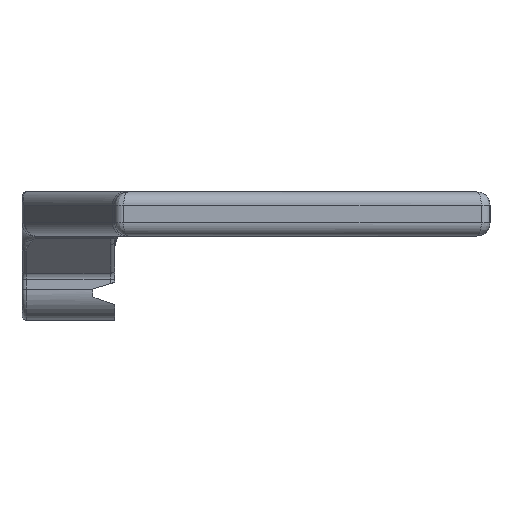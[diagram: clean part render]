
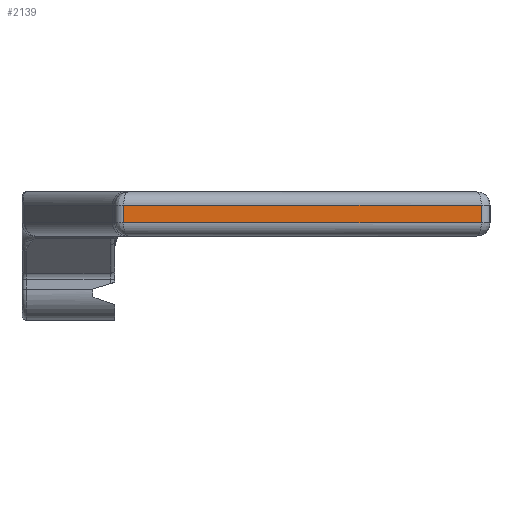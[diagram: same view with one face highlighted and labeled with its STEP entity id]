
A CAD part, left-side view. The second image highlights one B-rep face of the part: STEP entity #2139.
In plain terms, the highlighted planar face has unit normal (-1, 0, 0).
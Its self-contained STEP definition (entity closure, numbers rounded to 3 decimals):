
#67=PLANE('',#2383);
#225=FACE_OUTER_BOUND('',#368,.T.);
#368=EDGE_LOOP('',(#1737,#1738,#1739,#1740));
#515=LINE('',#4032,#679);
#524=LINE('',#4059,#688);
#525=LINE('',#4063,#689);
#526=LINE('',#4064,#690);
#679=VECTOR('',#2857,10.);
#688=VECTOR('',#2890,10.);
#689=VECTOR('',#2895,10.);
#690=VECTOR('',#2896,10.);
#1006=VERTEX_POINT('',#3931);
#1007=VERTEX_POINT('',#3965);
#1018=VERTEX_POINT('',#4058);
#1019=VERTEX_POINT('',#4062);
#1256=EDGE_CURVE('',#1006,#1007,#515,.T.);
#1269=EDGE_CURVE('',#1007,#1018,#524,.T.);
#1271=EDGE_CURVE('',#1019,#1006,#525,.T.);
#1272=EDGE_CURVE('',#1018,#1019,#526,.T.);
#1737=ORIENTED_EDGE('',*,*,#1256,.F.);
#1738=ORIENTED_EDGE('',*,*,#1271,.F.);
#1739=ORIENTED_EDGE('',*,*,#1272,.F.);
#1740=ORIENTED_EDGE('',*,*,#1269,.F.);
#2139=ADVANCED_FACE('',(#225),#67,.T.);
#2383=AXIS2_PLACEMENT_3D('',#4061,#2893,#2894);
#2857=DIRECTION('',(0.,-1.,0.));
#2890=DIRECTION('',(0.,0.,-1.));
#2893=DIRECTION('center_axis',(-1.,0.,0.));
#2894=DIRECTION('ref_axis',(0.,1.,0.));
#2895=DIRECTION('',(0.,0.,1.));
#2896=DIRECTION('',(0.,1.,0.));
#3931=CARTESIAN_POINT('',(-241.945,-9.43,-72.98));
#3965=CARTESIAN_POINT('',(-241.945,-90.43,-72.98));
#4032=CARTESIAN_POINT('',(-241.945,-68.68,-72.98));
#4058=CARTESIAN_POINT('',(-241.945,-90.43,-76.98));
#4059=CARTESIAN_POINT('',(-241.945,-90.43,-69.98));
#4061=CARTESIAN_POINT('Origin',(-241.945,-92.43,-69.98));
#4062=CARTESIAN_POINT('',(-241.945,-9.43,-76.98));
#4063=CARTESIAN_POINT('',(-241.945,-9.43,-69.98));
#4064=CARTESIAN_POINT('',(-241.945,-63.66,-76.98));
